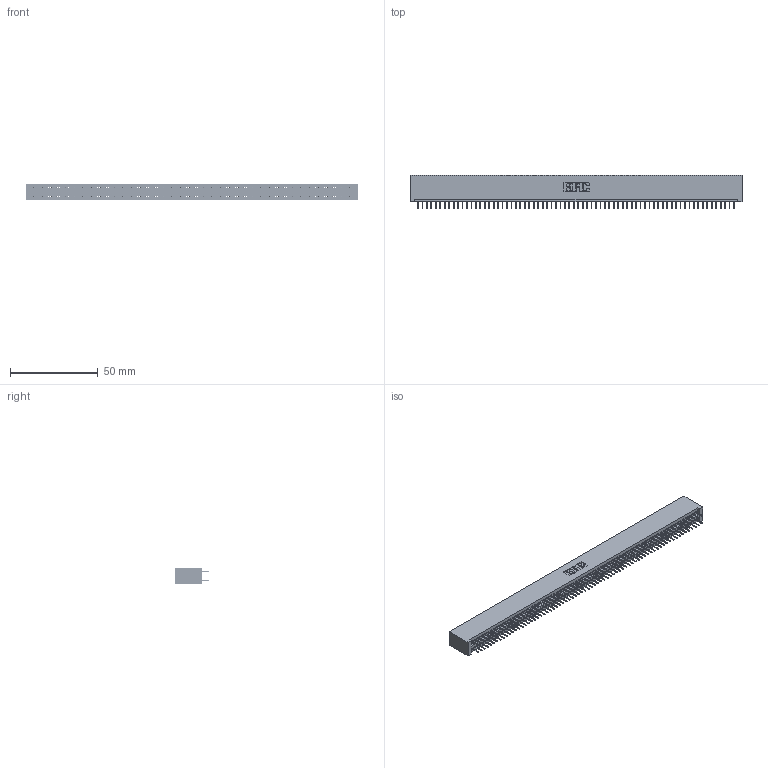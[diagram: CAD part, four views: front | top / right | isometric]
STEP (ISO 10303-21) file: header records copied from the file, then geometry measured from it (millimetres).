
FILE_DESCRIPTION (( 'STEP AP203' ), '1' );
FILE_NAME ('345-144-524-201.STEP', '2019-11-09T08:31:47', ( '' ), ( '' ), 'SwSTEP 2.0', 'SolidWorks 2016', '' );
FILE_SCHEMA (( 'CONFIG_CONTROL_DESIGN' ));
Length unit declared in the file: inch
Products named in the file (3): 345-292-001_345-293-124; 345 Part_No Mounting Lugs; 345-144-524-201
Assembly tree (145 placements, depth 2):
  345-144-524-201
    345 Part_No Mounting Lugs
    345-292-001_345-293-124  x144
Bounding box: 189.48 x 19.35 x 9.4 mm (x, y, z)
Volume: 19083.1 mm3; surface area: 28517.1 mm2
Topology: 145 solids, 145 shells, 7894 faces, 22349 edges, 14322 vertices
Faces by surface type: plane 5692, cylinder 2202
Entity records: 52251 total; most frequent: CARTESIAN_POINT 8728, ORIENTED_EDGE 8662, DIRECTION 7655, EDGE_CURVE 4331, VECTOR 3923, LINE 3923, VERTEX_POINT 2882, AXIS2_PLACEMENT_3D 1866
